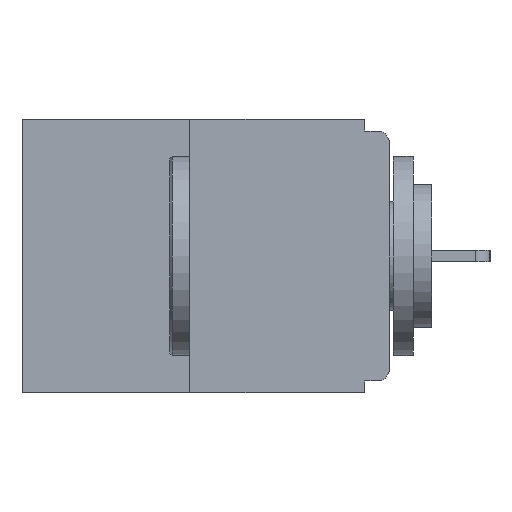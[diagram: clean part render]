
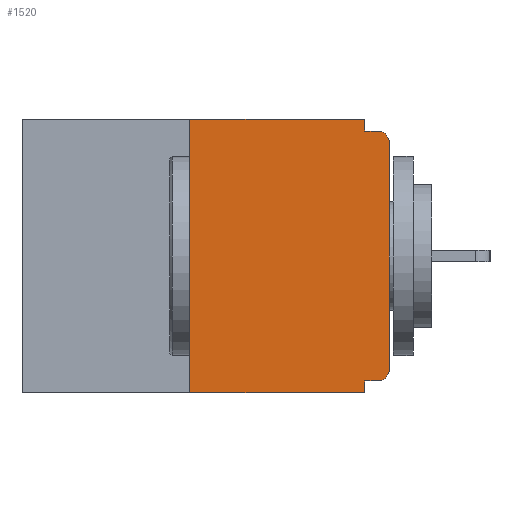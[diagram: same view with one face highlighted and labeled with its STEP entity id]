
A CAD part, left-side view. The second image highlights one B-rep face of the part: STEP entity #1520.
In plain terms, the highlighted planar face has unit normal (-1, 0, 0).
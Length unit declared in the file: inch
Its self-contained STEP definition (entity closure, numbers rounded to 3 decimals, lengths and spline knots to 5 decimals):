
#303 = EDGE_CURVE ( 'NONE', #1813, #13311, #3067, .T. ) ;
#597 = FACE_OUTER_BOUND ( 'NONE', #14084, .T. ) ;
#612 = VERTEX_POINT ( 'NONE', #12148 ) ;
#854 = DIRECTION ( 'NONE',  ( 1., 0., 0. ) ) ;
#1466 = DIRECTION ( 'NONE',  ( 0., -1., 0. ) ) ;
#1520 = ADVANCED_FACE ( 'NONE', ( #597 ), #15041, .F. ) ;
#1813 = VERTEX_POINT ( 'NONE', #14663 ) ;
#2128 = DIRECTION ( 'NONE',  ( 0., 0., -1. ) ) ;
#2476 = LINE ( 'NONE', #8013, #13587 ) ;
#3067 = LINE ( 'NONE', #7149, #9274 ) ;
#3085 = VERTEX_POINT ( 'NONE', #4634 ) ;
#3334 = ORIENTED_EDGE ( 'NONE', *, *, #10278, .F. ) ;
#3645 = EDGE_CURVE ( 'NONE', #12845, #13444, #8609, .T. ) ;
#3916 = CARTESIAN_POINT ( 'NONE',  ( 0., 0.015, -0.03 ) ) ;
#4009 = VECTOR ( 'NONE', #1466, 39.37008 ) ;
#4080 = VECTOR ( 'NONE', #16557, 39.37008 ) ;
#4367 = ORIENTED_EDGE ( 'NONE', *, *, #303, .F. ) ;
#4427 = DIRECTION ( 'NONE',  ( 0., 0., -1. ) ) ;
#4634 = CARTESIAN_POINT ( 'NONE',  ( 0., 0., -0.313 ) ) ;
#4661 = DIRECTION ( 'NONE',  ( 0., 0., 1. ) ) ;
#5613 = VECTOR ( 'NONE', #13201, 39.37008 ) ;
#5739 = VERTEX_POINT ( 'NONE', #16731 ) ;
#5770 = LINE ( 'NONE', #8600, #4080 ) ;
#5968 = LINE ( 'NONE', #13994, #15000 ) ;
#6405 = CARTESIAN_POINT ( 'NONE',  ( 0., 0.031, 0. ) ) ;
#6556 = DIRECTION ( 'NONE',  ( 0., -1., 0. ) ) ;
#6620 = LINE ( 'NONE', #13386, #5613 ) ;
#6701 = VERTEX_POINT ( 'NONE', #9775 ) ;
#6752 = ORIENTED_EDGE ( 'NONE', *, *, #9796, .T. ) ;
#7149 = CARTESIAN_POINT ( 'NONE',  ( 0., 0.25, 0. ) ) ;
#7772 = LINE ( 'NONE', #9231, #4009 ) ;
#8013 = CARTESIAN_POINT ( 'NONE',  ( 0., 0., -0.015 ) ) ;
#8131 = ORIENTED_EDGE ( 'NONE', *, *, #9115, .T. ) ;
#8349 = AXIS2_PLACEMENT_3D ( 'NONE', #14871, #14605, #4427 ) ;
#8388 = ORIENTED_EDGE ( 'NONE', *, *, #15516, .T. ) ;
#8600 = CARTESIAN_POINT ( 'NONE',  ( 0., 0., 0. ) ) ;
#8609 = CIRCLE ( 'NONE', #10792, 0.015 ) ;
#8719 = EDGE_CURVE ( 'NONE', #10786, #10632, #5968, .T. ) ;
#9046 = ORIENTED_EDGE ( 'NONE', *, *, #13167, .F. ) ;
#9115 = EDGE_CURVE ( 'NONE', #3085, #12845, #5770, .T. ) ;
#9231 = CARTESIAN_POINT ( 'NONE',  ( 0., 0.46, -0.343 ) ) ;
#9274 = VECTOR ( 'NONE', #4661, 39.37008 ) ;
#9552 = CARTESIAN_POINT ( 'NONE',  ( 0., 0.031, -0.015 ) ) ;
#9639 = DIRECTION ( 'NONE',  ( 0., 0., -1. ) ) ;
#9644 = ORIENTED_EDGE ( 'NONE', *, *, #8719, .F. ) ;
#9775 = CARTESIAN_POINT ( 'NONE',  ( 0., 0.015, -0.328 ) ) ;
#9796 = EDGE_CURVE ( 'NONE', #6701, #3085, #14071, .T. ) ;
#10035 = AXIS2_PLACEMENT_3D ( 'NONE', #12287, #854, #2128 ) ;
#10278 = EDGE_CURVE ( 'NONE', #612, #5739, #10933, .T. ) ;
#10294 = CARTESIAN_POINT ( 'NONE',  ( 0., 0.015, -0.015 ) ) ;
#10632 = VERTEX_POINT ( 'NONE', #9552 ) ;
#10786 = VERTEX_POINT ( 'NONE', #6405 ) ;
#10792 = AXIS2_PLACEMENT_3D ( 'NONE', #3916, #12817, #15320 ) ;
#10933 = LINE ( 'NONE', #12026, #12087 ) ;
#11162 = CARTESIAN_POINT ( 'NONE',  ( 0., 0.25, 0. ) ) ;
#11193 = DIRECTION ( 'NONE',  ( 0., 0., -1. ) ) ;
#11342 = CARTESIAN_POINT ( 'NONE',  ( 0., 0., -0.328 ) ) ;
#11542 = ORIENTED_EDGE ( 'NONE', *, *, #15902, .F. ) ;
#12026 = CARTESIAN_POINT ( 'NONE',  ( 0., 0.031, -0.343 ) ) ;
#12087 = VECTOR ( 'NONE', #9639, 39.37008 ) ;
#12148 = CARTESIAN_POINT ( 'NONE',  ( 0., 0.031, -0.328 ) ) ;
#12287 = CARTESIAN_POINT ( 'NONE',  ( 0., 0.46, 0. ) ) ;
#12817 = DIRECTION ( 'NONE',  ( -1., 0., 0. ) ) ;
#12845 = VERTEX_POINT ( 'NONE', #13570 ) ;
#13167 = EDGE_CURVE ( 'NONE', #13311, #10786, #6620, .T. ) ;
#13201 = DIRECTION ( 'NONE',  ( 0., -1., 0. ) ) ;
#13311 = VERTEX_POINT ( 'NONE', #11162 ) ;
#13386 = CARTESIAN_POINT ( 'NONE',  ( 0., 0.46, 0. ) ) ;
#13444 = VERTEX_POINT ( 'NONE', #10294 ) ;
#13570 = CARTESIAN_POINT ( 'NONE',  ( 0., 0., -0.03 ) ) ;
#13587 = VECTOR ( 'NONE', #6556, 39.37008 ) ;
#13806 = ORIENTED_EDGE ( 'NONE', *, *, #15866, .F. ) ;
#13994 = CARTESIAN_POINT ( 'NONE',  ( 0., 0.031, 0. ) ) ;
#13996 = LINE ( 'NONE', #11342, #16601 ) ;
#14071 = CIRCLE ( 'NONE', #8349, 0.015 ) ;
#14084 = EDGE_LOOP ( 'NONE', ( #9046, #4367, #8388, #3334, #13806, #6752, #8131, #14447, #11542, #9644 ) ) ;
#14447 = ORIENTED_EDGE ( 'NONE', *, *, #3645, .T. ) ;
#14605 = DIRECTION ( 'NONE',  ( -1., 0., 0. ) ) ;
#14663 = CARTESIAN_POINT ( 'NONE',  ( 0., 0.25, -0.343 ) ) ;
#14871 = CARTESIAN_POINT ( 'NONE',  ( 0., 0.015, -0.313 ) ) ;
#15000 = VECTOR ( 'NONE', #11193, 39.37008 ) ;
#15041 = PLANE ( 'NONE',  #10035 ) ;
#15320 = DIRECTION ( 'NONE',  ( 0., 0., -1. ) ) ;
#15516 = EDGE_CURVE ( 'NONE', #1813, #5739, #7772, .T. ) ;
#15866 = EDGE_CURVE ( 'NONE', #6701, #612, #13996, .T. ) ;
#15902 = EDGE_CURVE ( 'NONE', #10632, #13444, #2476, .T. ) ;
#16557 = DIRECTION ( 'NONE',  ( 0., 0., 1. ) ) ;
#16578 = DIRECTION ( 'NONE',  ( 0., 1., 0. ) ) ;
#16601 = VECTOR ( 'NONE', #16578, 39.37008 ) ;
#16731 = CARTESIAN_POINT ( 'NONE',  ( 0., 0.031, -0.343 ) ) ;
